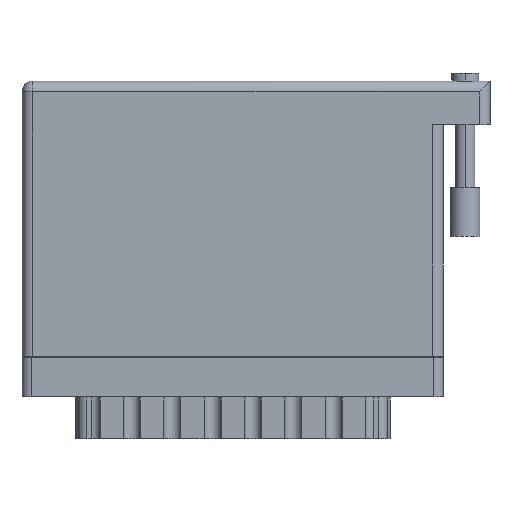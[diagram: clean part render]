
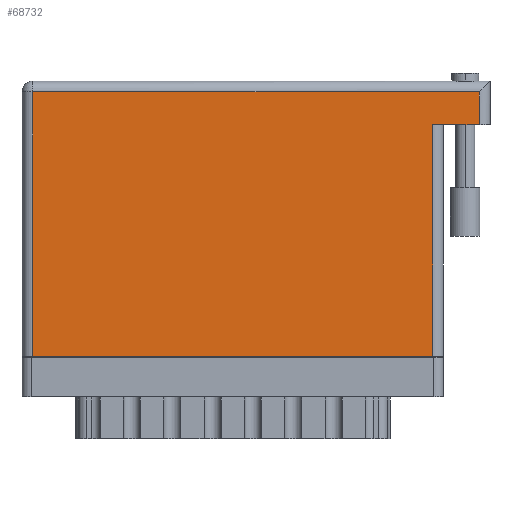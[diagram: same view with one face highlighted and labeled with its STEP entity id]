
A CAD part, front view. The second image highlights one B-rep face of the part: STEP entity #68732.
In plain terms, the highlighted face is planar.
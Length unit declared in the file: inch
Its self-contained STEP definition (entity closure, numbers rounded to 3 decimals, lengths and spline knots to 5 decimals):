
#1444 = EDGE_CURVE ( 'NONE', #12350, #44383, #10877, .T. ) ;
#1502 = CARTESIAN_POINT ( 'NONE',  ( 2.648, 1.495, 0. ) ) ;
#3763 = VECTOR ( 'NONE', #56848, 39.37008 ) ;
#6135 = AXIS2_PLACEMENT_3D ( 'NONE', #45575, #62338, #67069 ) ;
#6608 = CARTESIAN_POINT ( 'NONE',  ( 0.07, 0., 0. ) ) ;
#6792 = EDGE_CURVE ( 'NONE', #67023, #23492, #50587, .T. ) ;
#7143 = FACE_OUTER_BOUND ( 'NONE', #65676, .T. ) ;
#7659 = PLANE ( 'NONE',  #6135 ) ;
#9377 = ORIENTED_EDGE ( 'NONE', *, *, #60923, .F. ) ;
#10450 = VECTOR ( 'NONE', #21619, 39.37008 ) ;
#10877 = LINE ( 'NONE', #69144, #14282 ) ;
#11589 = ORIENTED_EDGE ( 'NONE', *, *, #1444, .T. ) ;
#11883 = ORIENTED_EDGE ( 'NONE', *, *, #62317, .T. ) ;
#12350 = VERTEX_POINT ( 'NONE', #30354 ) ;
#13529 = EDGE_CURVE ( 'NONE', #20767, #30036, #23243, .T. ) ;
#14282 = VECTOR ( 'NONE', #69859, 39.37008 ) ;
#14323 = DIRECTION ( 'NONE',  ( -1., 0., 0. ) ) ;
#14662 = CARTESIAN_POINT ( 'NONE',  ( 0.07, 1.705, 0. ) ) ;
#17590 = CARTESIAN_POINT ( 'NONE',  ( 0., 0., 0. ) ) ;
#20767 = VERTEX_POINT ( 'NONE', #48023 ) ;
#21619 = DIRECTION ( 'NONE',  ( 0., -1., 0. ) ) ;
#23243 = LINE ( 'NONE', #1502, #64344 ) ;
#23492 = VERTEX_POINT ( 'NONE', #6608 ) ;
#30036 = VERTEX_POINT ( 'NONE', #34544 ) ;
#30354 = CARTESIAN_POINT ( 'NONE',  ( 2.948, 1.495, 0. ) ) ;
#30677 = VECTOR ( 'NONE', #33603, 39.37008 ) ;
#32404 = LINE ( 'NONE', #17590, #30677 ) ;
#33603 = DIRECTION ( 'NONE',  ( 1., 0., 0. ) ) ;
#34544 = CARTESIAN_POINT ( 'NONE',  ( 2.648, 1.495, 0. ) ) ;
#42240 = CARTESIAN_POINT ( 'NONE',  ( 3.018, 1.495, 0. ) ) ;
#43047 = LINE ( 'NONE', #61861, #3763 ) ;
#43088 = CARTESIAN_POINT ( 'NONE',  ( 2.948, 1.705, 0. ) ) ;
#44383 = VERTEX_POINT ( 'NONE', #43088 ) ;
#45575 = CARTESIAN_POINT ( 'NONE',  ( 0., 1.775, 0. ) ) ;
#48023 = CARTESIAN_POINT ( 'NONE',  ( 2.648, 0., 0. ) ) ;
#48183 = ORIENTED_EDGE ( 'NONE', *, *, #13529, .T. ) ;
#50587 = LINE ( 'NONE', #60141, #10450 ) ;
#56848 = DIRECTION ( 'NONE',  ( -1., 0., 0. ) ) ;
#57372 = ORIENTED_EDGE ( 'NONE', *, *, #68701, .T. ) ;
#57460 = LINE ( 'NONE', #42240, #60007 ) ;
#60007 = VECTOR ( 'NONE', #14323, 39.37008 ) ;
#60141 = CARTESIAN_POINT ( 'NONE',  ( 0.07, 0., 0. ) ) ;
#60923 = EDGE_CURVE ( 'NONE', #12350, #30036, #57460, .T. ) ;
#61861 = CARTESIAN_POINT ( 'NONE',  ( 0., 1.705, 0. ) ) ;
#61958 = ORIENTED_EDGE ( 'NONE', *, *, #6792, .T. ) ;
#62317 = EDGE_CURVE ( 'NONE', #23492, #20767, #32404, .T. ) ;
#62338 = DIRECTION ( 'NONE',  ( 0., 0., -1. ) ) ;
#64344 = VECTOR ( 'NONE', #67320, 39.37008 ) ;
#65676 = EDGE_LOOP ( 'NONE', ( #11883, #48183, #9377, #11589, #57372, #61958 ) ) ;
#67023 = VERTEX_POINT ( 'NONE', #14662 ) ;
#67069 = DIRECTION ( 'NONE',  ( -1., 0., 0. ) ) ;
#67320 = DIRECTION ( 'NONE',  ( 0., 1., 0. ) ) ;
#68701 = EDGE_CURVE ( 'NONE', #44383, #67023, #43047, .T. ) ;
#68732 = ADVANCED_FACE ( 'NONE', ( #7143 ), #7659, .F. ) ;
#69144 = CARTESIAN_POINT ( 'NONE',  ( 2.948, 1.775, 0. ) ) ;
#69859 = DIRECTION ( 'NONE',  ( 0., 1., 0. ) ) ;
